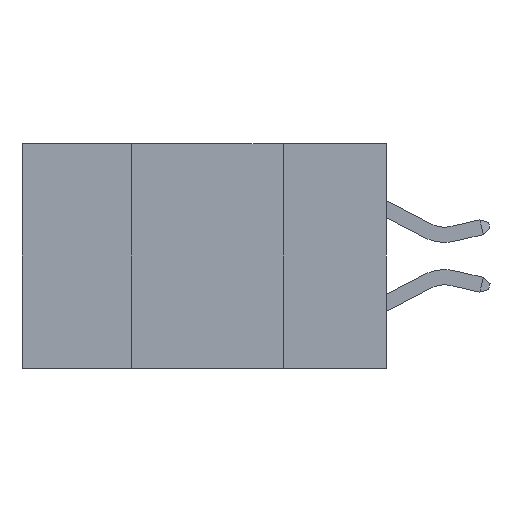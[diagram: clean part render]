
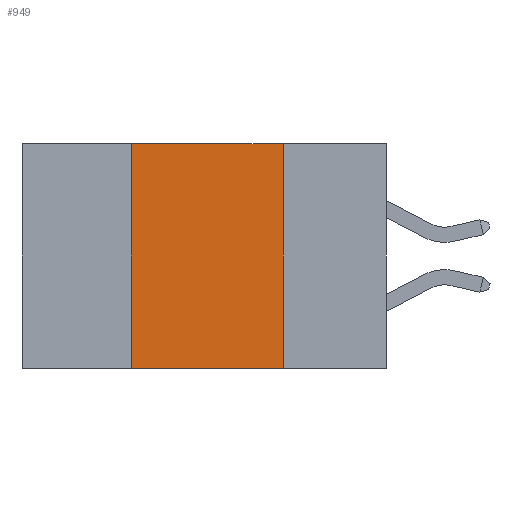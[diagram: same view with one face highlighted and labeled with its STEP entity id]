
A CAD part, left-side view. The second image highlights one B-rep face of the part: STEP entity #949.
In plain terms, the highlighted planar face has unit normal (-1, 0, 0).
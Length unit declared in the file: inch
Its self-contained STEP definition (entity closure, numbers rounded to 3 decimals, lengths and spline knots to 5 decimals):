
#58 = DIRECTION ( 'NONE',  ( 0., -1., 0. ) ) ;
#167 = CARTESIAN_POINT ( 'NONE',  ( 0., 0.6, 0. ) ) ;
#224 = CARTESIAN_POINT ( 'NONE',  ( 0., 0.42, -0.37 ) ) ;
#949 = ADVANCED_FACE ( 'NONE', ( #22972 ), #22865, .F. ) ;
#1938 = VECTOR ( 'NONE', #7737, 39.37008 ) ;
#2354 = CARTESIAN_POINT ( 'NONE',  ( 0., 0.6, -0.37 ) ) ;
#2520 = EDGE_CURVE ( 'NONE', #17146, #6364, #8182, .T. ) ;
#4007 = CARTESIAN_POINT ( 'NONE',  ( 0., 0.6, 0. ) ) ;
#6364 = VERTEX_POINT ( 'NONE', #18571 ) ;
#7245 = AXIS2_PLACEMENT_3D ( 'NONE', #4007, #16353, #20448 ) ;
#7737 = DIRECTION ( 'NONE',  ( 0., 0., -1. ) ) ;
#8182 = LINE ( 'NONE', #20388, #1938 ) ;
#8690 = ORIENTED_EDGE ( 'NONE', *, *, #2520, .F. ) ;
#10032 = ORIENTED_EDGE ( 'NONE', *, *, #16041, .T. ) ;
#10188 = VERTEX_POINT ( 'NONE', #21967 ) ;
#10204 = VECTOR ( 'NONE', #22760, 39.37008 ) ;
#10525 = VERTEX_POINT ( 'NONE', #224 ) ;
#10633 = VECTOR ( 'NONE', #58, 39.37008 ) ;
#14185 = LINE ( 'NONE', #2354, #10633 ) ;
#14961 = DIRECTION ( 'NONE',  ( 0., -1., 0. ) ) ;
#15241 = VECTOR ( 'NONE', #14961, 39.37008 ) ;
#15247 = EDGE_LOOP ( 'NONE', ( #8690, #19478, #22837, #10032 ) ) ;
#16041 = EDGE_CURVE ( 'NONE', #10525, #6364, #14185, .T. ) ;
#16353 = DIRECTION ( 'NONE',  ( 1., 0., 0. ) ) ;
#17146 = VERTEX_POINT ( 'NONE', #18876 ) ;
#18571 = CARTESIAN_POINT ( 'NONE',  ( 0., 0.17, -0.37 ) ) ;
#18876 = CARTESIAN_POINT ( 'NONE',  ( 0., 0.17, 0. ) ) ;
#19478 = ORIENTED_EDGE ( 'NONE', *, *, #20250, .F. ) ;
#20250 = EDGE_CURVE ( 'NONE', #10188, #17146, #21786, .T. ) ;
#20295 = LINE ( 'NONE', #27062, #10204 ) ;
#20388 = CARTESIAN_POINT ( 'NONE',  ( 0., 0.17, 0. ) ) ;
#20448 = DIRECTION ( 'NONE',  ( 0., 0., -1. ) ) ;
#21786 = LINE ( 'NONE', #167, #15241 ) ;
#21967 = CARTESIAN_POINT ( 'NONE',  ( 0., 0.42, 0. ) ) ;
#22698 = EDGE_CURVE ( 'NONE', #10525, #10188, #20295, .T. ) ;
#22760 = DIRECTION ( 'NONE',  ( 0., 0., 1. ) ) ;
#22837 = ORIENTED_EDGE ( 'NONE', *, *, #22698, .F. ) ;
#22865 = PLANE ( 'NONE',  #7245 ) ;
#22972 = FACE_OUTER_BOUND ( 'NONE', #15247, .T. ) ;
#27062 = CARTESIAN_POINT ( 'NONE',  ( 0., 0.42, 0. ) ) ;
